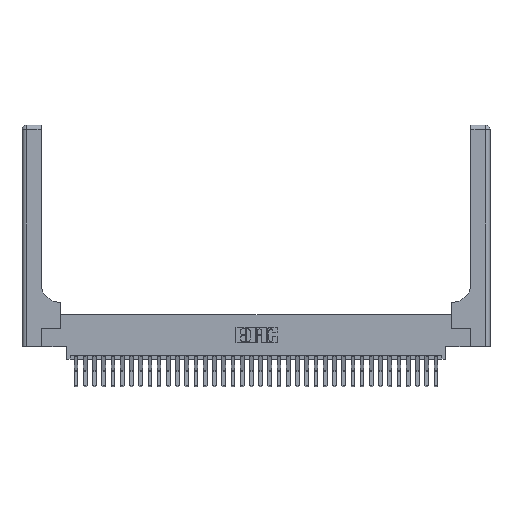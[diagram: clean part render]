
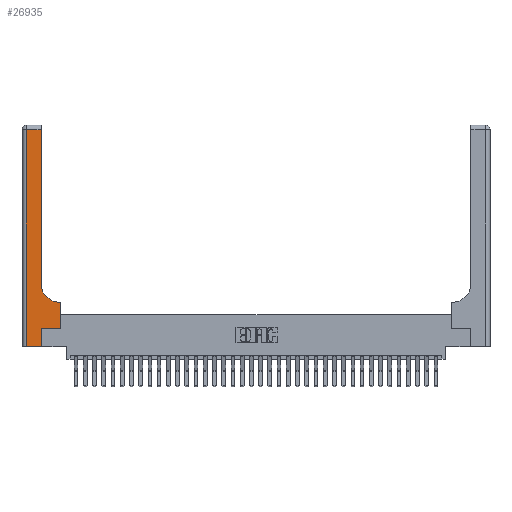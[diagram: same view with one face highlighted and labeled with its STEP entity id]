
A CAD part, top view. The second image highlights one B-rep face of the part: STEP entity #26935.
In plain terms, the highlighted planar face has unit normal (0, 0, 1).
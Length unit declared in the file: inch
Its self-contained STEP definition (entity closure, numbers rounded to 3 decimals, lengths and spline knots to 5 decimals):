
#194 = LINE ( 'NONE', #11426, #19142 ) ;
#468 = LINE ( 'NONE', #12467, #5558 ) ;
#769 = VECTOR ( 'NONE', #30252, 39.37008 ) ;
#874 = LINE ( 'NONE', #28138, #13289 ) ;
#1038 = CARTESIAN_POINT ( 'NONE',  ( 0.265, 0.25, 0.37 ) ) ;
#1111 = EDGE_CURVE ( 'NONE', #2066, #10797, #2634, .T. ) ;
#1578 = EDGE_CURVE ( 'NONE', #10797, #7531, #19171, .T. ) ;
#1581 = CARTESIAN_POINT ( 'NONE',  ( 0.26, 0.6, 0.37 ) ) ;
#1600 = VERTEX_POINT ( 'NONE', #5813 ) ;
#1830 = CARTESIAN_POINT ( 'NONE',  ( 0.51, 0.6, 0.37 ) ) ;
#2066 = VERTEX_POINT ( 'NONE', #29352 ) ;
#2135 = DIRECTION ( 'NONE',  ( 0., 0., -1. ) ) ;
#2634 = LINE ( 'NONE', #1581, #13479 ) ;
#3304 = LINE ( 'NONE', #11749, #8380 ) ;
#3416 = EDGE_CURVE ( 'NONE', #3987, #5652, #3304, .T. ) ;
#3980 = DIRECTION ( 'NONE',  ( -1., 0., 0. ) ) ;
#3987 = VERTEX_POINT ( 'NONE', #16426 ) ;
#4045 = DIRECTION ( 'NONE',  ( 0., -1., 0. ) ) ;
#4368 = EDGE_CURVE ( 'NONE', #29235, #1600, #13955, .T. ) ;
#5240 = VERTEX_POINT ( 'NONE', #7130 ) ;
#5346 = DIRECTION ( 'NONE',  ( 0., 1., 0. ) ) ;
#5506 = ORIENTED_EDGE ( 'NONE', *, *, #29932, .T. ) ;
#5558 = VECTOR ( 'NONE', #14926, 39.37008 ) ;
#5576 = ORIENTED_EDGE ( 'NONE', *, *, #1111, .T. ) ;
#5600 = AXIS2_PLACEMENT_3D ( 'NONE', #31496, #2135, #19394 ) ;
#5652 = VERTEX_POINT ( 'NONE', #6235 ) ;
#5813 = CARTESIAN_POINT ( 'NONE',  ( 0.528, 0.25, 0.37 ) ) ;
#6235 = CARTESIAN_POINT ( 'NONE',  ( 0.265, 0., 0.37 ) ) ;
#6345 = EDGE_CURVE ( 'NONE', #1600, #2066, #26825, .T. ) ;
#7130 = CARTESIAN_POINT ( 'NONE',  ( 0.26, 2.94, 0.37 ) ) ;
#7531 = VERTEX_POINT ( 'NONE', #29687 ) ;
#7850 = EDGE_CURVE ( 'NONE', #14374, #3987, #194, .T. ) ;
#8380 = VECTOR ( 'NONE', #16684, 39.37008 ) ;
#8602 = ORIENTED_EDGE ( 'NONE', *, *, #18878, .T. ) ;
#10797 = VERTEX_POINT ( 'NONE', #1830 ) ;
#11426 = CARTESIAN_POINT ( 'NONE',  ( 0.06, 3., 0.37 ) ) ;
#11749 = CARTESIAN_POINT ( 'NONE',  ( 0., 0., 0.37 ) ) ;
#11753 = EDGE_CURVE ( 'NONE', #5240, #14374, #468, .T. ) ;
#12467 = CARTESIAN_POINT ( 'NONE',  ( 0., 2.94, 0.37 ) ) ;
#12748 = ORIENTED_EDGE ( 'NONE', *, *, #4368, .T. ) ;
#13040 = ORIENTED_EDGE ( 'NONE', *, *, #11753, .T. ) ;
#13158 = CARTESIAN_POINT ( 'NONE',  ( 0.51, 0.85, 0.37 ) ) ;
#13289 = VECTOR ( 'NONE', #30541, 39.37008 ) ;
#13479 = VECTOR ( 'NONE', #3980, 39.37008 ) ;
#13955 = LINE ( 'NONE', #20473, #769 ) ;
#14374 = VERTEX_POINT ( 'NONE', #27285 ) ;
#14467 = PLANE ( 'NONE',  #5600 ) ;
#14926 = DIRECTION ( 'NONE',  ( -1., 0., 0. ) ) ;
#15632 = DIRECTION ( 'NONE',  ( 1., 0., 0. ) ) ;
#15704 = ORIENTED_EDGE ( 'NONE', *, *, #6345, .T. ) ;
#15713 = DIRECTION ( 'NONE',  ( 0., 1., 0. ) ) ;
#16426 = CARTESIAN_POINT ( 'NONE',  ( 0.06, 0., 0.37 ) ) ;
#16684 = DIRECTION ( 'NONE',  ( 1., 0., 0. ) ) ;
#17016 = EDGE_LOOP ( 'NONE', ( #5506, #13040, #25186, #19320, #8602, #12748, #15704, #5576, #30911 ) ) ;
#17603 = CARTESIAN_POINT ( 'NONE',  ( 0.528, 0.25, 0.37 ) ) ;
#17851 = VECTOR ( 'NONE', #15713, 39.37008 ) ;
#18223 = AXIS2_PLACEMENT_3D ( 'NONE', #13158, #30213, #15632 ) ;
#18878 = EDGE_CURVE ( 'NONE', #5652, #29235, #874, .T. ) ;
#19142 = VECTOR ( 'NONE', #4045, 39.37008 ) ;
#19171 = CIRCLE ( 'NONE', #18223, 0.25 ) ;
#19320 = ORIENTED_EDGE ( 'NONE', *, *, #3416, .T. ) ;
#19394 = DIRECTION ( 'NONE',  ( -1., 0., 0. ) ) ;
#20473 = CARTESIAN_POINT ( 'NONE',  ( 0.265, 0.25, 0.37 ) ) ;
#20628 = CARTESIAN_POINT ( 'NONE',  ( 0.26, 3., 0.37 ) ) ;
#22991 = FACE_OUTER_BOUND ( 'NONE', #17016, .T. ) ;
#24363 = LINE ( 'NONE', #20628, #17851 ) ;
#25186 = ORIENTED_EDGE ( 'NONE', *, *, #7850, .T. ) ;
#26069 = VECTOR ( 'NONE', #5346, 39.37008 ) ;
#26825 = LINE ( 'NONE', #17603, #26069 ) ;
#26935 = ADVANCED_FACE ( 'NONE', ( #22991 ), #14467, .F. ) ;
#27285 = CARTESIAN_POINT ( 'NONE',  ( 0.06, 2.94, 0.37 ) ) ;
#28138 = CARTESIAN_POINT ( 'NONE',  ( 0.265, 0., 0.37 ) ) ;
#29235 = VERTEX_POINT ( 'NONE', #1038 ) ;
#29352 = CARTESIAN_POINT ( 'NONE',  ( 0.528, 0.6, 0.37 ) ) ;
#29687 = CARTESIAN_POINT ( 'NONE',  ( 0.26, 0.85, 0.37 ) ) ;
#29932 = EDGE_CURVE ( 'NONE', #7531, #5240, #24363, .T. ) ;
#30213 = DIRECTION ( 'NONE',  ( 0., 0., -1. ) ) ;
#30252 = DIRECTION ( 'NONE',  ( 1., 0., 0. ) ) ;
#30541 = DIRECTION ( 'NONE',  ( 0., 1., 0. ) ) ;
#30911 = ORIENTED_EDGE ( 'NONE', *, *, #1578, .T. ) ;
#31496 = CARTESIAN_POINT ( 'NONE',  ( 0., 3., 0.37 ) ) ;
